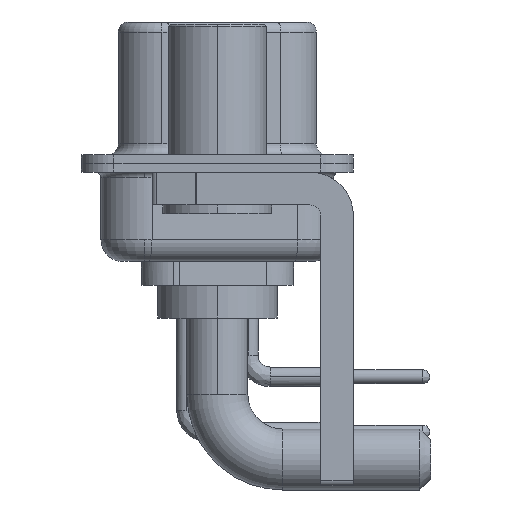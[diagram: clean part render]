
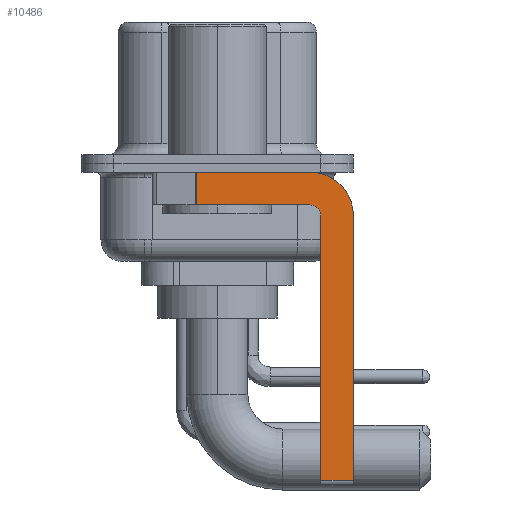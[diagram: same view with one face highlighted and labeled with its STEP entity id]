
A CAD part, left-side view. The second image highlights one B-rep face of the part: STEP entity #10486.
In plain terms, the highlighted planar face has unit normal (-1, 0, 0).
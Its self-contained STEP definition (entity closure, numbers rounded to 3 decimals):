
#171 = VERTEX_POINT ( 'NONE', #23644 ) ;
#533 = CARTESIAN_POINT ( 'NONE',  ( -2.9, -4.25, -1.9 ) ) ;
#955 = ORIENTED_EDGE ( 'NONE', *, *, #26588, .F. ) ;
#2180 = LINE ( 'NONE', #20954, #10934 ) ;
#2930 = LINE ( 'NONE', #25398, #10536 ) ;
#3776 = DIRECTION ( 'NONE',  ( 0., 0., 1. ) ) ;
#3839 = DIRECTION ( 'NONE',  ( 0., -1., 0. ) ) ;
#4823 = LINE ( 'NONE', #21923, #16876 ) ;
#5987 = CARTESIAN_POINT ( 'NONE',  ( -2.9, -4.25, -1.9 ) ) ;
#6318 = PLANE ( 'NONE',  #24537 ) ;
#6459 = DIRECTION ( 'NONE',  ( 0., 0., -1. ) ) ;
#6629 = ORIENTED_EDGE ( 'NONE', *, *, #24974, .F. ) ;
#6949 = ORIENTED_EDGE ( 'NONE', *, *, #26340, .F. ) ;
#7376 = VERTEX_POINT ( 'NONE', #25788 ) ;
#7394 = ORIENTED_EDGE ( 'NONE', *, *, #18417, .F. ) ;
#7583 = CARTESIAN_POINT ( 'NONE',  ( -2.9, -4.25, -0.4 ) ) ;
#7615 = VERTEX_POINT ( 'NONE', #12672 ) ;
#8009 = DIRECTION ( 'NONE',  ( 0., 0., -1. ) ) ;
#8707 = ORIENTED_EDGE ( 'NONE', *, *, #25717, .F. ) ;
#8712 = AXIS2_PLACEMENT_3D ( 'NONE', #12422, #14342, #8009 ) ;
#9097 = VERTEX_POINT ( 'NONE', #7583 ) ;
#10101 = EDGE_CURVE ( 'NONE', #7615, #9097, #17987, .T. ) ;
#10486 = ADVANCED_FACE ( 'NONE', ( #20679 ), #6318, .F. ) ;
#10536 = VECTOR ( 'NONE', #23344, 1000. ) ;
#10934 = VECTOR ( 'NONE', #3839, 1000. ) ;
#11768 = VERTEX_POINT ( 'NONE', #23733 ) ;
#12320 = EDGE_CURVE ( 'NONE', #7615, #171, #4823, .T. ) ;
#12422 = CARTESIAN_POINT ( 'NONE',  ( -2.9, -4.25, -2.4 ) ) ;
#12672 = CARTESIAN_POINT ( 'NONE',  ( -2.9, 0.978, -0.4 ) ) ;
#13251 = DIRECTION ( 'NONE',  ( 0., 0., -1. ) ) ;
#13342 = VERTEX_POINT ( 'NONE', #533 ) ;
#13854 = DIRECTION ( 'NONE',  ( 0., -1., 0. ) ) ;
#14342 = DIRECTION ( 'NONE',  ( 1., 0., 0. ) ) ;
#14488 = AXIS2_PLACEMENT_3D ( 'NONE', #24993, #14677, #3776 ) ;
#14677 = DIRECTION ( 'NONE',  ( -1., 0., 0. ) ) ;
#15070 = LINE ( 'NONE', #21260, #21566 ) ;
#15912 = CARTESIAN_POINT ( 'NONE',  ( -2.9, 3., -0.4 ) ) ;
#16876 = VECTOR ( 'NONE', #13251, 1000. ) ;
#17117 = VECTOR ( 'NONE', #24730, 1000. ) ;
#17987 = LINE ( 'NONE', #15912, #23687 ) ;
#18417 = EDGE_CURVE ( 'NONE', #9097, #7376, #24524, .T. ) ;
#18882 = DIRECTION ( 'NONE',  ( 1., 0., 0. ) ) ;
#18982 = VERTEX_POINT ( 'NONE', #26687 ) ;
#20679 = FACE_OUTER_BOUND ( 'NONE', #26299, .T. ) ;
#20954 = CARTESIAN_POINT ( 'NONE',  ( -2.9, -4.25, -14.55 ) ) ;
#21240 = ORIENTED_EDGE ( 'NONE', *, *, #12320, .T. ) ;
#21260 = CARTESIAN_POINT ( 'NONE',  ( -2.9, -4.75, -14.8 ) ) ;
#21566 = VECTOR ( 'NONE', #23955, 1000. ) ;
#21923 = CARTESIAN_POINT ( 'NONE',  ( -2.9, 0.978, -1.9 ) ) ;
#22478 = ORIENTED_EDGE ( 'NONE', *, *, #24081, .T. ) ;
#22582 = CARTESIAN_POINT ( 'NONE',  ( -2.9, -4.25, -2.4 ) ) ;
#23143 = CARTESIAN_POINT ( 'NONE',  ( -2.9, -4.75, -2.4 ) ) ;
#23344 = DIRECTION ( 'NONE',  ( 0., 0., -1. ) ) ;
#23377 = VERTEX_POINT ( 'NONE', #23143 ) ;
#23644 = CARTESIAN_POINT ( 'NONE',  ( -2.9, 0.978, -1.9 ) ) ;
#23687 = VECTOR ( 'NONE', #13854, 1000. ) ;
#23733 = CARTESIAN_POINT ( 'NONE',  ( -2.9, -6.25, -14.55 ) ) ;
#23955 = DIRECTION ( 'NONE',  ( 0., 0., 1. ) ) ;
#24081 = EDGE_CURVE ( 'NONE', #18982, #11768, #2180, .T. ) ;
#24524 = CIRCLE ( 'NONE', #8712, 2. ) ;
#24537 = AXIS2_PLACEMENT_3D ( 'NONE', #22582, #18882, #6459 ) ;
#24730 = DIRECTION ( 'NONE',  ( 0., 1., 0. ) ) ;
#24974 = EDGE_CURVE ( 'NONE', #23377, #13342, #26337, .T. ) ;
#24993 = CARTESIAN_POINT ( 'NONE',  ( -2.9, -4.25, -2.4 ) ) ;
#25356 = ORIENTED_EDGE ( 'NONE', *, *, #10101, .F. ) ;
#25398 = CARTESIAN_POINT ( 'NONE',  ( -2.9, -6.25, -2.4 ) ) ;
#25717 = EDGE_CURVE ( 'NONE', #18982, #23377, #15070, .T. ) ;
#25788 = CARTESIAN_POINT ( 'NONE',  ( -2.9, -6.25, -2.4 ) ) ;
#26299 = EDGE_LOOP ( 'NONE', ( #25356, #21240, #6949, #6629, #8707, #22478, #955, #7394 ) ) ;
#26337 = CIRCLE ( 'NONE', #14488, 0.5 ) ;
#26340 = EDGE_CURVE ( 'NONE', #13342, #171, #26926, .T. ) ;
#26588 = EDGE_CURVE ( 'NONE', #7376, #11768, #2930, .T. ) ;
#26687 = CARTESIAN_POINT ( 'NONE',  ( -2.9, -4.75, -14.55 ) ) ;
#26926 = LINE ( 'NONE', #5987, #17117 ) ;
